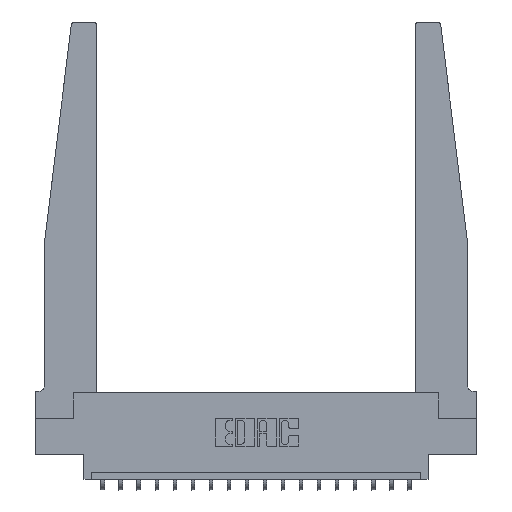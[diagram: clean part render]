
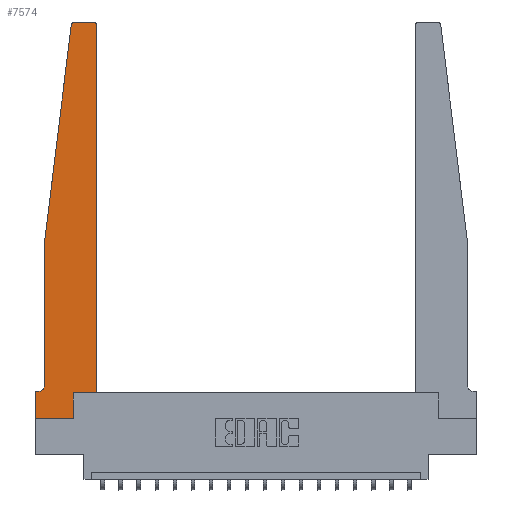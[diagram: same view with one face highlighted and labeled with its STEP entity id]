
A CAD part, top view. The second image highlights one B-rep face of the part: STEP entity #7574.
In plain terms, the highlighted planar face has unit normal (0, 0, 1).
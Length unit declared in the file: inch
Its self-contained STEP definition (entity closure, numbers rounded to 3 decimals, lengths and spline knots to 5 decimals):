
#119 = EDGE_CURVE ( 'NONE', #10550, #2545, #7658, .T. ) ;
#144 = LINE ( 'NONE', #14665, #11605 ) ;
#176 = ORIENTED_EDGE ( 'NONE', *, *, #8260, .T. ) ;
#550 = DIRECTION ( 'NONE',  ( -1., 0., 0. ) ) ;
#767 = EDGE_CURVE ( 'NONE', #9390, #14340, #4188, .T. ) ;
#804 = CARTESIAN_POINT ( 'NONE',  ( 0.015, 0.1875, 0.37 ) ) ;
#990 = EDGE_CURVE ( 'NONE', #11670, #6132, #13252, .T. ) ;
#1323 = CIRCLE ( 'NONE', #8870, 0.03 ) ;
#2093 = DIRECTION ( 'NONE',  ( 0., 1., 0. ) ) ;
#2291 = ORIENTED_EDGE ( 'NONE', *, *, #990, .T. ) ;
#2545 = VERTEX_POINT ( 'NONE', #11665 ) ;
#2552 = EDGE_CURVE ( 'NONE', #14340, #12989, #7429, .T. ) ;
#2648 = CARTESIAN_POINT ( 'NONE',  ( 0.425, 0.18, 0.37 ) ) ;
#2675 = EDGE_LOOP ( 'NONE', ( #5360, #13735, #17720, #2291, #18666, #7207, #11633, #176, #6513, #16539, #4861, #9253 ) ) ;
#2744 = CARTESIAN_POINT ( 'NONE',  ( 0.25, 2.75, 0.37 ) ) ;
#2933 = CARTESIAN_POINT ( 'NONE',  ( 0.065, 0.2375, 0.37 ) ) ;
#3486 = VECTOR ( 'NONE', #4263, 39.37008 ) ;
#3672 = EDGE_CURVE ( 'NONE', #8975, #9390, #4392, .T. ) ;
#4101 = AXIS2_PLACEMENT_3D ( 'NONE', #16651, #10513, #5316 ) ;
#4188 = CIRCLE ( 'NONE', #4101, 0.03 ) ;
#4263 = DIRECTION ( 'NONE',  ( -1., 0., 0. ) ) ;
#4392 = LINE ( 'NONE', #15923, #8335 ) ;
#4861 = ORIENTED_EDGE ( 'NONE', *, *, #3672, .T. ) ;
#4921 = AXIS2_PLACEMENT_3D ( 'NONE', #14489, #5579, #15981 ) ;
#5316 = DIRECTION ( 'NONE',  ( 1., 0., 0. ) ) ;
#5360 = ORIENTED_EDGE ( 'NONE', *, *, #2552, .T. ) ;
#5462 = CIRCLE ( 'NONE', #6918, 0.05 ) ;
#5519 = CARTESIAN_POINT ( 'NONE',  ( 0.395, 2.75, 0.37 ) ) ;
#5552 = CARTESIAN_POINT ( 'NONE',  ( 0.2605, 0.18, 0.37 ) ) ;
#5579 = DIRECTION ( 'NONE',  ( 0., 0., 1. ) ) ;
#5756 = DIRECTION ( 'NONE',  ( 1., 0., 0. ) ) ;
#6132 = VERTEX_POINT ( 'NONE', #2933 ) ;
#6444 = VERTEX_POINT ( 'NONE', #5552 ) ;
#6513 = ORIENTED_EDGE ( 'NONE', *, *, #7384, .T. ) ;
#6918 = AXIS2_PLACEMENT_3D ( 'NONE', #18469, #9495, #550 ) ;
#7006 = DIRECTION ( 'NONE',  ( 0., 1., 0. ) ) ;
#7195 = VECTOR ( 'NONE', #9423, 39.37008 ) ;
#7207 = ORIENTED_EDGE ( 'NONE', *, *, #119, .T. ) ;
#7270 = LINE ( 'NONE', #11040, #11234 ) ;
#7341 = DIRECTION ( 'NONE',  ( 0., -1., 0. ) ) ;
#7384 = EDGE_CURVE ( 'NONE', #18188, #6444, #7270, .T. ) ;
#7429 = LINE ( 'NONE', #2744, #3486 ) ;
#7550 = DIRECTION ( 'NONE',  ( 0., 0., 1. ) ) ;
#7574 = ADVANCED_FACE ( 'NONE', ( #11914 ), #11481, .T. ) ;
#7658 = LINE ( 'NONE', #14388, #7195 ) ;
#7952 = VERTEX_POINT ( 'NONE', #10874 ) ;
#8225 = CARTESIAN_POINT ( 'NONE',  ( 0.065, 1.25, 0.37 ) ) ;
#8260 = EDGE_CURVE ( 'NONE', #16769, #18188, #8628, .T. ) ;
#8335 = VECTOR ( 'NONE', #7006, 39.37008 ) ;
#8628 = LINE ( 'NONE', #16088, #16095 ) ;
#8870 = AXIS2_PLACEMENT_3D ( 'NONE', #16479, #7550, #18006 ) ;
#8975 = VERTEX_POINT ( 'NONE', #2648 ) ;
#9253 = ORIENTED_EDGE ( 'NONE', *, *, #767, .T. ) ;
#9390 = VERTEX_POINT ( 'NONE', #14239 ) ;
#9423 = DIRECTION ( 'NONE',  ( -1., 0., 0. ) ) ;
#9495 = DIRECTION ( 'NONE',  ( 0., 0., -1. ) ) ;
#10513 = DIRECTION ( 'NONE',  ( 0., 0., 1. ) ) ;
#10550 = VERTEX_POINT ( 'NONE', #804 ) ;
#10874 = CARTESIAN_POINT ( 'NONE',  ( 0.24675, 2.72367, 0.37 ) ) ;
#11000 = VECTOR ( 'NONE', #7341, 39.37008 ) ;
#11040 = CARTESIAN_POINT ( 'NONE',  ( 0.2605, 0.18, 0.37 ) ) ;
#11234 = VECTOR ( 'NONE', #2093, 39.37008 ) ;
#11286 = CARTESIAN_POINT ( 'NONE',  ( 0.2605, 0., 0.37 ) ) ;
#11462 = LINE ( 'NONE', #13261, #11000 ) ;
#11481 = PLANE ( 'NONE',  #4921 ) ;
#11605 = VECTOR ( 'NONE', #5756, 39.37008 ) ;
#11633 = ORIENTED_EDGE ( 'NONE', *, *, #14812, .T. ) ;
#11656 = DIRECTION ( 'NONE',  ( 1., 0., 0. ) ) ;
#11665 = CARTESIAN_POINT ( 'NONE',  ( 0., 0.1875, 0.37 ) ) ;
#11670 = VERTEX_POINT ( 'NONE', #13962 ) ;
#11914 = FACE_OUTER_BOUND ( 'NONE', #2675, .T. ) ;
#12319 = VECTOR ( 'NONE', #13807, 39.37008 ) ;
#12989 = VERTEX_POINT ( 'NONE', #18817 ) ;
#13252 = LINE ( 'NONE', #16808, #12319 ) ;
#13261 = CARTESIAN_POINT ( 'NONE',  ( 0., 0., 0.37 ) ) ;
#13735 = ORIENTED_EDGE ( 'NONE', *, *, #16121, .T. ) ;
#13807 = DIRECTION ( 'NONE',  ( 0., -1., 0. ) ) ;
#13962 = CARTESIAN_POINT ( 'NONE',  ( 0.065, 1.25, 0.37 ) ) ;
#14142 = VECTOR ( 'NONE', #17169, 39.37008 ) ;
#14239 = CARTESIAN_POINT ( 'NONE',  ( 0.425, 2.72, 0.37 ) ) ;
#14340 = VERTEX_POINT ( 'NONE', #5519 ) ;
#14388 = CARTESIAN_POINT ( 'NONE',  ( 0.065, 0.1875, 0.37 ) ) ;
#14489 = CARTESIAN_POINT ( 'NONE',  ( 0., 0.1875, 0.37 ) ) ;
#14665 = CARTESIAN_POINT ( 'NONE',  ( 0.425, 0.18, 0.37 ) ) ;
#14812 = EDGE_CURVE ( 'NONE', #2545, #16769, #11462, .T. ) ;
#15923 = CARTESIAN_POINT ( 'NONE',  ( 0.425, 0.18, 0.37 ) ) ;
#15950 = EDGE_CURVE ( 'NONE', #6444, #8975, #144, .T. ) ;
#15981 = DIRECTION ( 'NONE',  ( 1., 0., 0. ) ) ;
#16088 = CARTESIAN_POINT ( 'NONE',  ( 0., 0., 0.37 ) ) ;
#16095 = VECTOR ( 'NONE', #11656, 39.37008 ) ;
#16121 = EDGE_CURVE ( 'NONE', #12989, #7952, #1323, .T. ) ;
#16479 = CARTESIAN_POINT ( 'NONE',  ( 0.27653, 2.72, 0.37 ) ) ;
#16539 = ORIENTED_EDGE ( 'NONE', *, *, #15950, .T. ) ;
#16651 = CARTESIAN_POINT ( 'NONE',  ( 0.395, 2.72, 0.37 ) ) ;
#16769 = VERTEX_POINT ( 'NONE', #18048 ) ;
#16808 = CARTESIAN_POINT ( 'NONE',  ( 0.065, 1.25, 0.37 ) ) ;
#17017 = EDGE_CURVE ( 'NONE', #7952, #11670, #17649, .T. ) ;
#17169 = DIRECTION ( 'NONE',  ( -0.122, -0.992, 0. ) ) ;
#17649 = LINE ( 'NONE', #8225, #14142 ) ;
#17720 = ORIENTED_EDGE ( 'NONE', *, *, #17017, .T. ) ;
#18006 = DIRECTION ( 'NONE',  ( 1., 0., 0. ) ) ;
#18048 = CARTESIAN_POINT ( 'NONE',  ( 0., 0., 0.37 ) ) ;
#18188 = VERTEX_POINT ( 'NONE', #11286 ) ;
#18469 = CARTESIAN_POINT ( 'NONE',  ( 0.015, 0.2375, 0.37 ) ) ;
#18666 = ORIENTED_EDGE ( 'NONE', *, *, #18668, .T. ) ;
#18668 = EDGE_CURVE ( 'NONE', #6132, #10550, #5462, .T. ) ;
#18817 = CARTESIAN_POINT ( 'NONE',  ( 0.27653, 2.75, 0.37 ) ) ;
